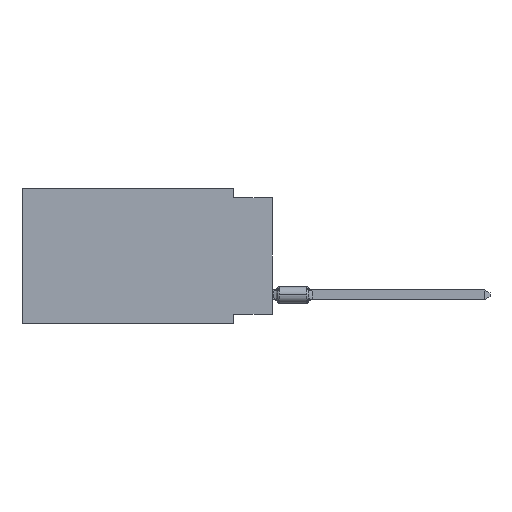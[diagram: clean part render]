
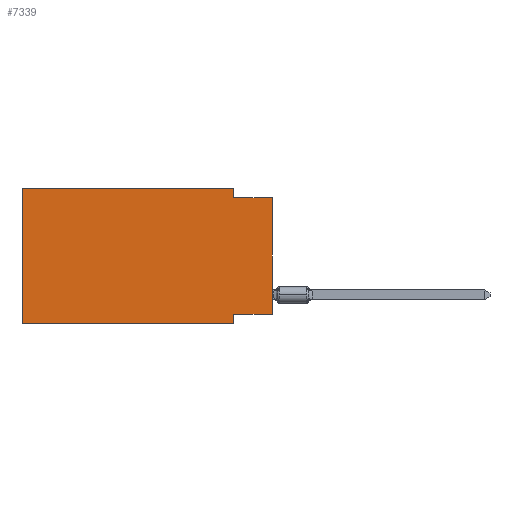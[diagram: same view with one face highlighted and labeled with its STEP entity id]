
A CAD part, left-side view. The second image highlights one B-rep face of the part: STEP entity #7339.
In plain terms, the highlighted planar face has unit normal (-1, 0, 0).
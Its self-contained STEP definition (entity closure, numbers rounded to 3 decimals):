
#244 = AXIS2_PLACEMENT_3D ( 'NONE', #15693, #15814, #1038 ) ;
#978 = ORIENTED_EDGE ( 'NONE', *, *, #17694, .F. ) ;
#1038 = DIRECTION ( 'NONE',  ( 0., 0., -1. ) ) ;
#1584 = VERTEX_POINT ( 'NONE', #6487 ) ;
#1646 = CARTESIAN_POINT ( 'NONE',  ( 0., 2.54, 0. ) ) ;
#1668 = LINE ( 'NONE', #20707, #16001 ) ;
#1689 = EDGE_CURVE ( 'NONE', #6192, #18563, #12925, .T. ) ;
#1833 = EDGE_CURVE ( 'NONE', #20962, #3986, #21397, .T. ) ;
#2226 = DIRECTION ( 'NONE',  ( 0., 1., 0. ) ) ;
#2489 = VERTEX_POINT ( 'NONE', #5370 ) ;
#2741 = EDGE_LOOP ( 'NONE', ( #19099, #17889, #11390, #11503, #4794, #22656, #978, #4568 ) ) ;
#3284 = VERTEX_POINT ( 'NONE', #22127 ) ;
#3986 = VERTEX_POINT ( 'NONE', #6301 ) ;
#4010 = DIRECTION ( 'NONE',  ( 0., 0., 1. ) ) ;
#4384 = VECTOR ( 'NONE', #18543, 1000. ) ;
#4405 = VECTOR ( 'NONE', #4010, 1000. ) ;
#4568 = ORIENTED_EDGE ( 'NONE', *, *, #1833, .F. ) ;
#4794 = ORIENTED_EDGE ( 'NONE', *, *, #9077, .F. ) ;
#5370 = CARTESIAN_POINT ( 'NONE',  ( 0., 16.383, 0. ) ) ;
#5569 = DIRECTION ( 'NONE',  ( 0., 0., -1. ) ) ;
#5571 = CARTESIAN_POINT ( 'NONE',  ( 0., 0., -0.635 ) ) ;
#5910 = CARTESIAN_POINT ( 'NONE',  ( 0., 2.54, -8.89 ) ) ;
#6192 = VERTEX_POINT ( 'NONE', #16521 ) ;
#6301 = CARTESIAN_POINT ( 'NONE',  ( 0., 2.54, -8.255 ) ) ;
#6487 = CARTESIAN_POINT ( 'NONE',  ( 0., 2.54, -0.635 ) ) ;
#7339 = ADVANCED_FACE ( 'NONE', ( #14079 ), #21578, .F. ) ;
#7472 = CARTESIAN_POINT ( 'NONE',  ( 0., 0., 0. ) ) ;
#7793 = VERTEX_POINT ( 'NONE', #5571 ) ;
#7941 = CARTESIAN_POINT ( 'NONE',  ( 0., 16.383, 0. ) ) ;
#8229 = LINE ( 'NONE', #14119, #22868 ) ;
#8578 = EDGE_CURVE ( 'NONE', #20962, #7793, #11292, .T. ) ;
#9077 = EDGE_CURVE ( 'NONE', #6192, #2489, #13716, .T. ) ;
#9178 = VECTOR ( 'NONE', #5569, 1000. ) ;
#9416 = DIRECTION ( 'NONE',  ( 0., -1., 0. ) ) ;
#10099 = EDGE_CURVE ( 'NONE', #1584, #7793, #8229, .T. ) ;
#10146 = VECTOR ( 'NONE', #10973, 1000. ) ;
#10973 = DIRECTION ( 'NONE',  ( 0., -1., 0. ) ) ;
#11074 = EDGE_CURVE ( 'NONE', #3284, #1584, #22653, .T. ) ;
#11292 = LINE ( 'NONE', #7472, #4384 ) ;
#11390 = ORIENTED_EDGE ( 'NONE', *, *, #11074, .F. ) ;
#11503 = ORIENTED_EDGE ( 'NONE', *, *, #21647, .F. ) ;
#11797 = CARTESIAN_POINT ( 'NONE',  ( 0., 0., -8.255 ) ) ;
#12925 = LINE ( 'NONE', #18459, #10146 ) ;
#13276 = VECTOR ( 'NONE', #2226, 1000. ) ;
#13716 = LINE ( 'NONE', #7941, #4405 ) ;
#14079 = FACE_OUTER_BOUND ( 'NONE', #2741, .T. ) ;
#14119 = CARTESIAN_POINT ( 'NONE',  ( 0., 0., -0.635 ) ) ;
#14982 = CARTESIAN_POINT ( 'NONE',  ( 0., 2.54, -8.89 ) ) ;
#15693 = CARTESIAN_POINT ( 'NONE',  ( 0., 16.383, 0. ) ) ;
#15741 = DIRECTION ( 'NONE',  ( 0., -1., 0. ) ) ;
#15814 = DIRECTION ( 'NONE',  ( 1., 0., 0. ) ) ;
#16001 = VECTOR ( 'NONE', #9416, 1000. ) ;
#16521 = CARTESIAN_POINT ( 'NONE',  ( 0., 16.383, -8.89 ) ) ;
#17694 = EDGE_CURVE ( 'NONE', #3986, #18563, #24306, .T. ) ;
#17889 = ORIENTED_EDGE ( 'NONE', *, *, #10099, .F. ) ;
#18459 = CARTESIAN_POINT ( 'NONE',  ( 0., 16.383, -8.89 ) ) ;
#18543 = DIRECTION ( 'NONE',  ( 0., 0., 1. ) ) ;
#18563 = VERTEX_POINT ( 'NONE', #5910 ) ;
#19099 = ORIENTED_EDGE ( 'NONE', *, *, #8578, .T. ) ;
#20707 = CARTESIAN_POINT ( 'NONE',  ( 0., 16.383, 0. ) ) ;
#20962 = VERTEX_POINT ( 'NONE', #11797 ) ;
#21152 = CARTESIAN_POINT ( 'NONE',  ( 0., 0., -8.255 ) ) ;
#21397 = LINE ( 'NONE', #21152, #13276 ) ;
#21578 = PLANE ( 'NONE',  #244 ) ;
#21647 = EDGE_CURVE ( 'NONE', #2489, #3284, #1668, .T. ) ;
#22127 = CARTESIAN_POINT ( 'NONE',  ( 0., 2.54, 0. ) ) ;
#22481 = DIRECTION ( 'NONE',  ( 0., 0., -1. ) ) ;
#22653 = LINE ( 'NONE', #1646, #9178 ) ;
#22656 = ORIENTED_EDGE ( 'NONE', *, *, #1689, .T. ) ;
#22868 = VECTOR ( 'NONE', #15741, 1000. ) ;
#23500 = VECTOR ( 'NONE', #22481, 1000. ) ;
#24306 = LINE ( 'NONE', #14982, #23500 ) ;
